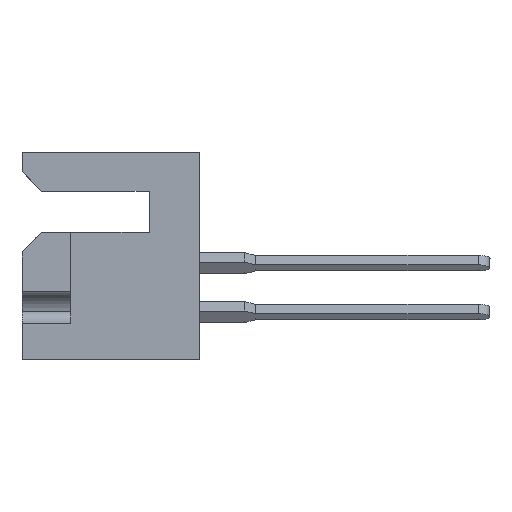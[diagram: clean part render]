
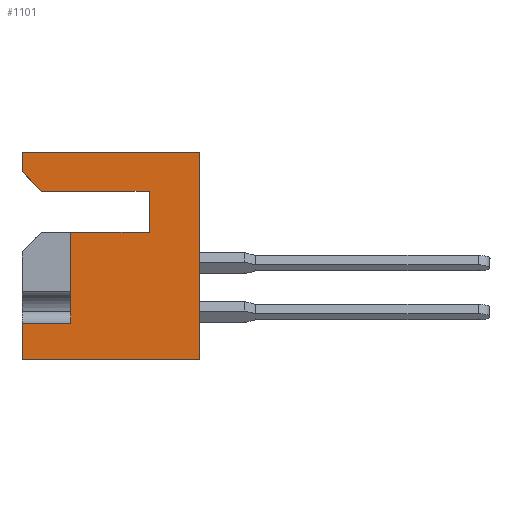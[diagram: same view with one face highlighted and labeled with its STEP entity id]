
A CAD part, left-side view. The second image highlights one B-rep face of the part: STEP entity #1101.
In plain terms, the highlighted planar face has unit normal (-1, 0, 0).
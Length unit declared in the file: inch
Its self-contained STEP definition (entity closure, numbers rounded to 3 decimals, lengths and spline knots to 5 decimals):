
#533 = CARTESIAN_POINT ( 'NONE',  ( 0., 0.453, -0.437 ) ) ;
#697 = DIRECTION ( 'NONE',  ( 0., 0., 1. ) ) ;
#785 = DIRECTION ( 'NONE',  ( 0., -1., 0. ) ) ;
#1101 = ADVANCED_FACE ( 'NONE', ( #22008 ), #11069, .F. ) ;
#1794 = DIRECTION ( 'NONE',  ( 0., 0., 1. ) ) ;
#2142 = ORIENTED_EDGE ( 'NONE', *, *, #11244, .F. ) ;
#2545 = CARTESIAN_POINT ( 'NONE',  ( 0., 0.403, -0.1 ) ) ;
#3085 = VECTOR ( 'NONE', #697, 39.37008 ) ;
#3114 = VERTEX_POINT ( 'NONE', #11413 ) ;
#3462 = CARTESIAN_POINT ( 'NONE',  ( 0., 0.453, -0.05 ) ) ;
#4533 = VECTOR ( 'NONE', #13536, 39.37008 ) ;
#4886 = DIRECTION ( 'NONE',  ( 0., -1., 0. ) ) ;
#5017 = CARTESIAN_POINT ( 'NONE',  ( 0., 0.128, -0.205 ) ) ;
#5081 = EDGE_CURVE ( 'NONE', #21369, #3114, #13436, .T. ) ;
#5103 = VECTOR ( 'NONE', #8989, 39.37008 ) ;
#5144 = ORIENTED_EDGE ( 'NONE', *, *, #24995, .T. ) ;
#5744 = EDGE_CURVE ( 'NONE', #21369, #23789, #7852, .T. ) ;
#5778 = EDGE_CURVE ( 'NONE', #19374, #16455, #12759, .T. ) ;
#6588 = CARTESIAN_POINT ( 'NONE',  ( 0., 0.453, -0.531 ) ) ;
#6774 = DIRECTION ( 'NONE',  ( 0., -0.707, -0.707 ) ) ;
#6852 = CARTESIAN_POINT ( 'NONE',  ( 0., 0.328, -0.205 ) ) ;
#7458 = CARTESIAN_POINT ( 'NONE',  ( 0., 0.328, -0.205 ) ) ;
#7540 = CARTESIAN_POINT ( 'NONE',  ( 0., 0., -0.531 ) ) ;
#7852 = LINE ( 'NONE', #2545, #23946 ) ;
#7991 = LINE ( 'NONE', #16194, #17489 ) ;
#8527 = VECTOR ( 'NONE', #25011, 39.37008 ) ;
#8605 = EDGE_CURVE ( 'NONE', #19374, #25798, #14223, .T. ) ;
#8877 = EDGE_CURVE ( 'NONE', #15592, #17037, #7991, .T. ) ;
#8989 = DIRECTION ( 'NONE',  ( 0., 1., 0. ) ) ;
#10031 = CARTESIAN_POINT ( 'NONE',  ( 0., 0.453, 0. ) ) ;
#10074 = DIRECTION ( 'NONE',  ( 0., 0., 1. ) ) ;
#10461 = VECTOR ( 'NONE', #785, 39.37008 ) ;
#10547 = VECTOR ( 'NONE', #4886, 39.37008 ) ;
#10884 = CARTESIAN_POINT ( 'NONE',  ( 0., 0.453, 0. ) ) ;
#10990 = LINE ( 'NONE', #19572, #26770 ) ;
#11069 = PLANE ( 'NONE',  #13971 ) ;
#11244 = EDGE_CURVE ( 'NONE', #3114, #15222, #21632, .T. ) ;
#11378 = DIRECTION ( 'NONE',  ( 0., 0., 1. ) ) ;
#11413 = CARTESIAN_POINT ( 'NONE',  ( 0., 0.453, 0. ) ) ;
#11543 = CARTESIAN_POINT ( 'NONE',  ( 0., 0.453, 0. ) ) ;
#12759 = LINE ( 'NONE', #5017, #4533 ) ;
#13021 = CARTESIAN_POINT ( 'NONE',  ( 0., 0.328, -0.437 ) ) ;
#13372 = CARTESIAN_POINT ( 'NONE',  ( 0., 0.128, -0.1 ) ) ;
#13436 = LINE ( 'NONE', #10031, #8527 ) ;
#13536 = DIRECTION ( 'NONE',  ( 0., 1., 0. ) ) ;
#13971 = AXIS2_PLACEMENT_3D ( 'NONE', #10884, #19308, #23569 ) ;
#14223 = LINE ( 'NONE', #13372, #22476 ) ;
#14350 = ORIENTED_EDGE ( 'NONE', *, *, #5081, .F. ) ;
#14595 = VECTOR ( 'NONE', #10074, 39.37008 ) ;
#15053 = DIRECTION ( 'NONE',  ( 0., 1., 0. ) ) ;
#15222 = VERTEX_POINT ( 'NONE', #22218 ) ;
#15592 = VERTEX_POINT ( 'NONE', #6588 ) ;
#15896 = ORIENTED_EDGE ( 'NONE', *, *, #8877, .F. ) ;
#16106 = LINE ( 'NONE', #17540, #10547 ) ;
#16194 = CARTESIAN_POINT ( 'NONE',  ( 0., 0.453, 0. ) ) ;
#16241 = LINE ( 'NONE', #21573, #5103 ) ;
#16298 = EDGE_CURVE ( 'NONE', #25798, #23789, #10990, .T. ) ;
#16455 = VERTEX_POINT ( 'NONE', #7458 ) ;
#16708 = ORIENTED_EDGE ( 'NONE', *, *, #5744, .T. ) ;
#16856 = VERTEX_POINT ( 'NONE', #13021 ) ;
#17028 = EDGE_CURVE ( 'NONE', #16856, #17037, #16241, .T. ) ;
#17037 = VERTEX_POINT ( 'NONE', #533 ) ;
#17489 = VECTOR ( 'NONE', #1794, 39.37008 ) ;
#17493 = ORIENTED_EDGE ( 'NONE', *, *, #16298, .F. ) ;
#17540 = CARTESIAN_POINT ( 'NONE',  ( 0., 0.453, -0.531 ) ) ;
#18527 = ORIENTED_EDGE ( 'NONE', *, *, #5778, .T. ) ;
#18909 = ORIENTED_EDGE ( 'NONE', *, *, #24143, .T. ) ;
#19308 = DIRECTION ( 'NONE',  ( 1., 0., 0. ) ) ;
#19374 = VERTEX_POINT ( 'NONE', #26029 ) ;
#19572 = CARTESIAN_POINT ( 'NONE',  ( 0., 0.128, -0.1 ) ) ;
#19721 = ORIENTED_EDGE ( 'NONE', *, *, #17028, .T. ) ;
#20086 = VERTEX_POINT ( 'NONE', #7540 ) ;
#21193 = ORIENTED_EDGE ( 'NONE', *, *, #8605, .F. ) ;
#21369 = VERTEX_POINT ( 'NONE', #3462 ) ;
#21458 = EDGE_LOOP ( 'NONE', ( #19721, #15896, #18909, #5144, #2142, #14350, #16708, #17493, #21193, #18527, #26529 ) ) ;
#21573 = CARTESIAN_POINT ( 'NONE',  ( 0., 0.328, -0.437 ) ) ;
#21632 = LINE ( 'NONE', #11543, #10461 ) ;
#22008 = FACE_OUTER_BOUND ( 'NONE', #21458, .T. ) ;
#22145 = LINE ( 'NONE', #6852, #3085 ) ;
#22218 = CARTESIAN_POINT ( 'NONE',  ( 0., 0., 0. ) ) ;
#22309 = CARTESIAN_POINT ( 'NONE',  ( 0., 0., 0. ) ) ;
#22476 = VECTOR ( 'NONE', #11378, 39.37008 ) ;
#23569 = DIRECTION ( 'NONE',  ( 0., 0., -1. ) ) ;
#23789 = VERTEX_POINT ( 'NONE', #24289 ) ;
#23946 = VECTOR ( 'NONE', #6774, 39.37008 ) ;
#24143 = EDGE_CURVE ( 'NONE', #15592, #20086, #16106, .T. ) ;
#24187 = CARTESIAN_POINT ( 'NONE',  ( 0., 0.128, -0.1 ) ) ;
#24289 = CARTESIAN_POINT ( 'NONE',  ( 0., 0.403, -0.1 ) ) ;
#24806 = LINE ( 'NONE', #22309, #14595 ) ;
#24995 = EDGE_CURVE ( 'NONE', #20086, #15222, #24806, .T. ) ;
#25011 = DIRECTION ( 'NONE',  ( 0., 0., 1. ) ) ;
#25499 = EDGE_CURVE ( 'NONE', #16856, #16455, #22145, .T. ) ;
#25798 = VERTEX_POINT ( 'NONE', #24187 ) ;
#26029 = CARTESIAN_POINT ( 'NONE',  ( 0., 0.128, -0.205 ) ) ;
#26529 = ORIENTED_EDGE ( 'NONE', *, *, #25499, .F. ) ;
#26770 = VECTOR ( 'NONE', #15053, 39.37008 ) ;
